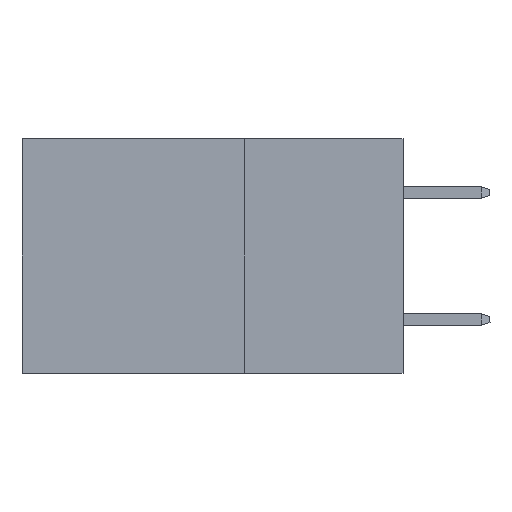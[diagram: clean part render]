
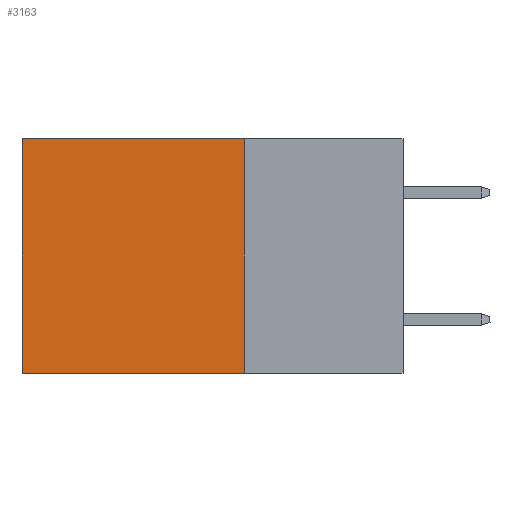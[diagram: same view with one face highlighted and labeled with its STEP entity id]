
A CAD part, left-side view. The second image highlights one B-rep face of the part: STEP entity #3163.
In plain terms, the highlighted planar face has unit normal (-1, 0, 0).
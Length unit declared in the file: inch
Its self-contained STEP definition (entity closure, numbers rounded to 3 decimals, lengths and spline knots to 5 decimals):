
#89 = FACE_OUTER_BOUND ( 'NONE', #12261, .T. ) ;
#463 = VECTOR ( 'NONE', #9395, 39.37008 ) ;
#814 = CARTESIAN_POINT ( 'NONE',  ( 0.2875, 0.25, 0. ) ) ;
#1330 = CARTESIAN_POINT ( 'NONE',  ( 0.2875, 0.6, -0.37 ) ) ;
#1575 = DIRECTION ( 'NONE',  ( 0., 0., -1. ) ) ;
#2863 = LINE ( 'NONE', #5944, #10790 ) ;
#3163 = ADVANCED_FACE ( 'NONE', ( #89 ), #7663, .F. ) ;
#3498 = VERTEX_POINT ( 'NONE', #3702 ) ;
#3688 = VECTOR ( 'NONE', #1575, 39.37008 ) ;
#3702 = CARTESIAN_POINT ( 'NONE',  ( 0.2875, 0.6, 0. ) ) ;
#3709 = VERTEX_POINT ( 'NONE', #1330 ) ;
#3863 = EDGE_CURVE ( 'NONE', #13062, #3498, #11670, .T. ) ;
#4127 = AXIS2_PLACEMENT_3D ( 'NONE', #8655, #10970, #10048 ) ;
#4373 = EDGE_CURVE ( 'NONE', #3498, #3709, #13556, .T. ) ;
#5132 = VECTOR ( 'NONE', #9836, 39.37008 ) ;
#5944 = CARTESIAN_POINT ( 'NONE',  ( 0.2875, 0.25, 0. ) ) ;
#6238 = CARTESIAN_POINT ( 'NONE',  ( 0.2875, 0.25, 0. ) ) ;
#6741 = VERTEX_POINT ( 'NONE', #9284 ) ;
#7273 = DIRECTION ( 'NONE',  ( 0., 0., -1. ) ) ;
#7663 = PLANE ( 'NONE',  #4127 ) ;
#8205 = ORIENTED_EDGE ( 'NONE', *, *, #4373, .T. ) ;
#8655 = CARTESIAN_POINT ( 'NONE',  ( 0.2875, 0.25, 0. ) ) ;
#8856 = LINE ( 'NONE', #11895, #5132 ) ;
#9284 = CARTESIAN_POINT ( 'NONE',  ( 0.2875, 0.25, -0.37 ) ) ;
#9395 = DIRECTION ( 'NONE',  ( 0., 1., 0. ) ) ;
#9486 = EDGE_CURVE ( 'NONE', #13062, #6741, #2863, .T. ) ;
#9836 = DIRECTION ( 'NONE',  ( 0., 1., 0. ) ) ;
#10048 = DIRECTION ( 'NONE',  ( 0., 0., -1. ) ) ;
#10149 = ORIENTED_EDGE ( 'NONE', *, *, #3863, .T. ) ;
#10790 = VECTOR ( 'NONE', #7273, 39.37008 ) ;
#10880 = EDGE_CURVE ( 'NONE', #6741, #3709, #8856, .T. ) ;
#10970 = DIRECTION ( 'NONE',  ( 1., 0., 0. ) ) ;
#11499 = ORIENTED_EDGE ( 'NONE', *, *, #9486, .F. ) ;
#11670 = LINE ( 'NONE', #6238, #463 ) ;
#11895 = CARTESIAN_POINT ( 'NONE',  ( 0.2875, 0.25, -0.37 ) ) ;
#12261 = EDGE_LOOP ( 'NONE', ( #8205, #12761, #11499, #10149 ) ) ;
#12391 = CARTESIAN_POINT ( 'NONE',  ( 0.2875, 0.6, 0. ) ) ;
#12761 = ORIENTED_EDGE ( 'NONE', *, *, #10880, .F. ) ;
#13062 = VERTEX_POINT ( 'NONE', #814 ) ;
#13556 = LINE ( 'NONE', #12391, #3688 ) ;
